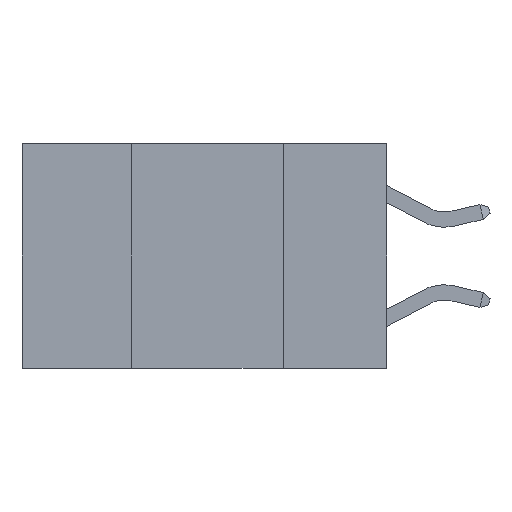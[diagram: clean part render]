
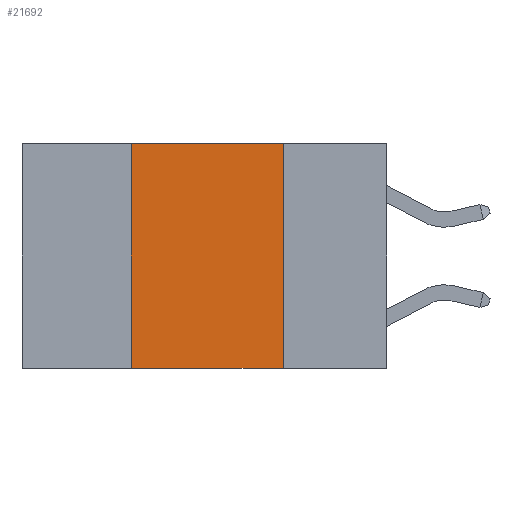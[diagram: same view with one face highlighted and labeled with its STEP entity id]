
A CAD part, left-side view. The second image highlights one B-rep face of the part: STEP entity #21692.
In plain terms, the highlighted planar face has unit normal (-1, 0, 0).
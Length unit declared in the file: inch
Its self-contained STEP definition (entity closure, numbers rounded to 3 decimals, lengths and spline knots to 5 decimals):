
#390 = VERTEX_POINT ( 'NONE', #4649 ) ;
#1181 = ORIENTED_EDGE ( 'NONE', *, *, #18843, .T. ) ;
#2266 = CARTESIAN_POINT ( 'NONE',  ( 0., 0.6, -0.37 ) ) ;
#3151 = DIRECTION ( 'NONE',  ( 1., 0., 0. ) ) ;
#3717 = CARTESIAN_POINT ( 'NONE',  ( 0., 0.42, 0. ) ) ;
#4649 = CARTESIAN_POINT ( 'NONE',  ( 0., 0.17, -0.37 ) ) ;
#5219 = EDGE_CURVE ( 'NONE', #20757, #18506, #21998, .T. ) ;
#6280 = VECTOR ( 'NONE', #19083, 39.37008 ) ;
#6654 = LINE ( 'NONE', #18247, #8325 ) ;
#8251 = DIRECTION ( 'NONE',  ( 0., -1., 0. ) ) ;
#8325 = VECTOR ( 'NONE', #8803, 39.37008 ) ;
#8803 = DIRECTION ( 'NONE',  ( 0., 0., -1. ) ) ;
#9957 = DIRECTION ( 'NONE',  ( 0., -1., 0. ) ) ;
#13277 = AXIS2_PLACEMENT_3D ( 'NONE', #14236, #3151, #24183 ) ;
#13842 = LINE ( 'NONE', #2266, #22423 ) ;
#14236 = CARTESIAN_POINT ( 'NONE',  ( 0., 0.6, 0. ) ) ;
#15218 = LINE ( 'NONE', #3717, #6280 ) ;
#18247 = CARTESIAN_POINT ( 'NONE',  ( 0., 0.17, 0. ) ) ;
#18371 = PLANE ( 'NONE',  #13277 ) ;
#18448 = EDGE_CURVE ( 'NONE', #21812, #20757, #15218, .T. ) ;
#18506 = VERTEX_POINT ( 'NONE', #21744 ) ;
#18746 = CARTESIAN_POINT ( 'NONE',  ( 0., 0.42, -0.37 ) ) ;
#18843 = EDGE_CURVE ( 'NONE', #21812, #390, #13842, .T. ) ;
#18986 = EDGE_CURVE ( 'NONE', #18506, #390, #6654, .T. ) ;
#19083 = DIRECTION ( 'NONE',  ( 0., 0., 1. ) ) ;
#19702 = CARTESIAN_POINT ( 'NONE',  ( 0., 0.6, 0. ) ) ;
#20075 = CARTESIAN_POINT ( 'NONE',  ( 0., 0.42, 0. ) ) ;
#20757 = VERTEX_POINT ( 'NONE', #20075 ) ;
#21692 = ADVANCED_FACE ( 'NONE', ( #22181 ), #18371, .F. ) ;
#21744 = CARTESIAN_POINT ( 'NONE',  ( 0., 0.17, 0. ) ) ;
#21812 = VERTEX_POINT ( 'NONE', #18746 ) ;
#21917 = EDGE_LOOP ( 'NONE', ( #24259, #22538, #24202, #1181 ) ) ;
#21998 = LINE ( 'NONE', #19702, #22442 ) ;
#22181 = FACE_OUTER_BOUND ( 'NONE', #21917, .T. ) ;
#22423 = VECTOR ( 'NONE', #9957, 39.37008 ) ;
#22442 = VECTOR ( 'NONE', #8251, 39.37008 ) ;
#22538 = ORIENTED_EDGE ( 'NONE', *, *, #5219, .F. ) ;
#24183 = DIRECTION ( 'NONE',  ( 0., 0., -1. ) ) ;
#24202 = ORIENTED_EDGE ( 'NONE', *, *, #18448, .F. ) ;
#24259 = ORIENTED_EDGE ( 'NONE', *, *, #18986, .F. ) ;
